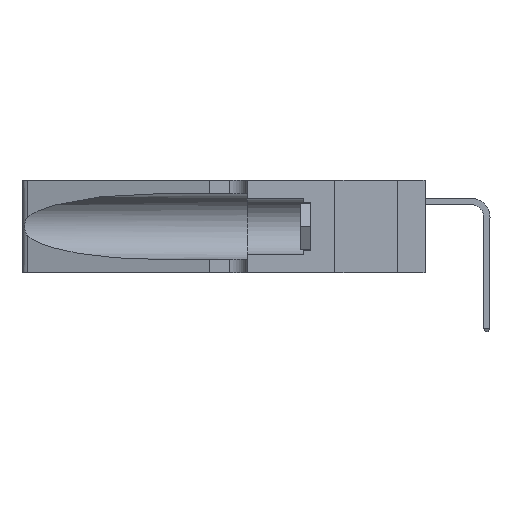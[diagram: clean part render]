
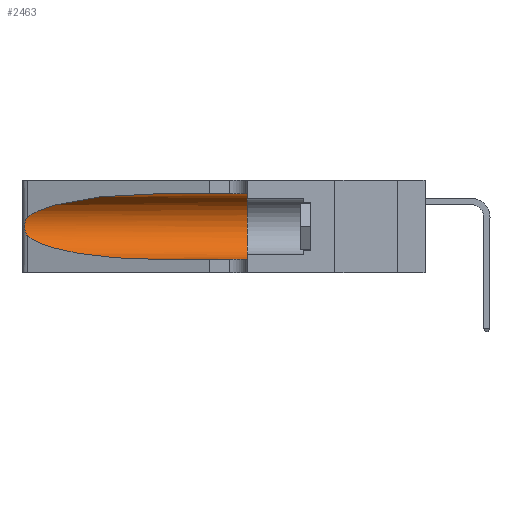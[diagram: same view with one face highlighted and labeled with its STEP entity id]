
A CAD part, left-side view. The second image highlights one B-rep face of the part: STEP entity #2463.
In plain terms, the highlighted cylindrical face has radius 3.308 mm (diameter 6.617 mm), a partial arc.
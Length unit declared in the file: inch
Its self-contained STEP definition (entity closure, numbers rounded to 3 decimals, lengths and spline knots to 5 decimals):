
#19 = EDGE_CURVE ( 'NONE', #4897, #9281, #9336, .T. ) ;
#1151 = CARTESIAN_POINT ( 'NONE',  ( 0.1305, 0.72297, 0.31525 ) ) ;
#1165 = EDGE_CURVE ( 'NONE', #18363, #14374, #10308, .T. ) ;
#2083 = CARTESIAN_POINT ( 'NONE',  ( 0.25487, 1.22718, 0.14631 ) ) ;
#2425 = VECTOR ( 'NONE', #9149, 39.37008 ) ;
#2463 = ADVANCED_FACE ( 'NONE', ( #28487 ), #27783, .F. ) ;
#2698 =( BOUNDED_CURVE ( )  B_SPLINE_CURVE ( 3, ( #21450, #7989, #10233, #25913 ),
 .UNSPECIFIED., .F., .T. ) 
 B_SPLINE_CURVE_WITH_KNOTS ( ( 4, 4 ),
 ( 3.44316, 4.71239 ),
 .UNSPECIFIED. ) 
 CURVE ( )  GEOMETRIC_REPRESENTATION_ITEM ( )  RATIONAL_B_SPLINE_CURVE ( ( 1., 0.87, 0.87, 1. ) ) 
 REPRESENTATION_ITEM ( '' )  );
#3135 = LINE ( 'NONE', #20375, #2425 ) ;
#4897 = VERTEX_POINT ( 'NONE', #9453 ) ;
#5233 = ORIENTED_EDGE ( 'NONE', *, *, #1165, .T. ) ;
#5377 = CARTESIAN_POINT ( 'NONE',  ( 0.25787, 1.23484, 0.2124 ) ) ;
#5499 = CARTESIAN_POINT ( 'NONE',  ( 0.26018, 1.23835, 0.19895 ) ) ;
#6035 = CARTESIAN_POINT ( 'NONE',  ( 0.25487, 1.22718, 0.22369 ) ) ;
#6212 = CARTESIAN_POINT ( 'NONE',  ( 0.1305, 0.35, 0.05475 ) ) ;
#6290 = DIRECTION ( 'NONE',  ( 0., 1., 0. ) ) ;
#6357 = ORIENTED_EDGE ( 'NONE', *, *, #15109, .T. ) ;
#7962 = CARTESIAN_POINT ( 'NONE',  ( 0.2373, 1.15595, 0.28018 ) ) ;
#7989 = CARTESIAN_POINT ( 'NONE',  ( 0.2373, 1.15595, 0.08982 ) ) ;
#8105 = EDGE_CURVE ( 'NONE', #29033, #28754, #3135, .T. ) ;
#8364 = DIRECTION ( 'NONE',  ( 0., -1., 0. ) ) ;
#9149 = DIRECTION ( 'NONE',  ( 0., -1., 0. ) ) ;
#9281 = VERTEX_POINT ( 'NONE', #2083 ) ;
#9336 = B_SPLINE_CURVE_WITH_KNOTS ( 'NONE', 3,
 ( #6035, #24203, #21112, #5377, #25054, #5499, #20204, #19311, #28400, #12207, #18271, #28893, #12236, #26032 ),
 .UNSPECIFIED., .F., .F.,
 ( 4, 2, 2, 2, 2, 2, 4 ),
 ( 0., 0.00027, 0.00053, 0.00107, 0.0016, 0.00187, 0.00214 ),
 .UNSPECIFIED. ) ;
#9420 = CARTESIAN_POINT ( 'NONE',  ( 0.1305, 0.35, 0.31525 ) ) ;
#9453 = CARTESIAN_POINT ( 'NONE',  ( 0.25487, 1.22718, 0.22369 ) ) ;
#10233 = CARTESIAN_POINT ( 'NONE',  ( 0.18966, 0.96281, 0.05475 ) ) ;
#10308 = LINE ( 'NONE', #19622, #16332 ) ;
#10312 = AXIS2_PLACEMENT_3D ( 'NONE', #19779, #6290, #22014 ) ;
#10639 = DIRECTION ( 'NONE',  ( 0., 0., -1. ) ) ;
#10972 =( BOUNDED_CURVE ( )  B_SPLINE_CURVE ( 3, ( #1151, #14653, #7962, #23666 ),
 .UNSPECIFIED., .F., .F. ) 
 B_SPLINE_CURVE_WITH_KNOTS ( ( 4, 4 ),
 ( 1.5708, 2.84003 ),
 .UNSPECIFIED. ) 
 CURVE ( )  GEOMETRIC_REPRESENTATION_ITEM ( )  RATIONAL_B_SPLINE_CURVE ( ( 1., 0.87, 0.87, 1. ) ) 
 REPRESENTATION_ITEM ( '' )  );
#11423 = AXIS2_PLACEMENT_3D ( 'NONE', #19651, #21858, #10639 ) ;
#12207 = CARTESIAN_POINT ( 'NONE',  ( 0.25856, 1.23593, 0.16098 ) ) ;
#12236 = CARTESIAN_POINT ( 'NONE',  ( 0.25555, 1.22993, 0.14849 ) ) ;
#12429 = ORIENTED_EDGE ( 'NONE', *, *, #8105, .F. ) ;
#14333 = ORIENTED_EDGE ( 'NONE', *, *, #19, .T. ) ;
#14374 = VERTEX_POINT ( 'NONE', #6212 ) ;
#14653 = CARTESIAN_POINT ( 'NONE',  ( 0.18966, 0.96281, 0.31525 ) ) ;
#15109 = EDGE_CURVE ( 'NONE', #9281, #18363, #2698, .T. ) ;
#15769 = CARTESIAN_POINT ( 'NONE',  ( 0.1305, 0.72297, 0.05475 ) ) ;
#16332 = VECTOR ( 'NONE', #8364, 39.37008 ) ;
#17617 = EDGE_CURVE ( 'NONE', #29033, #4897, #10972, .T. ) ;
#17755 = EDGE_LOOP ( 'NONE', ( #17910, #14333, #6357, #5233, #22226, #12429 ) ) ;
#17910 = ORIENTED_EDGE ( 'NONE', *, *, #17617, .T. ) ;
#18271 = CARTESIAN_POINT ( 'NONE',  ( 0.25789, 1.23486, 0.15765 ) ) ;
#18363 = VERTEX_POINT ( 'NONE', #15769 ) ;
#18863 = EDGE_CURVE ( 'NONE', #28754, #14374, #26099, .T. ) ;
#19311 = CARTESIAN_POINT ( 'NONE',  ( 0.26075, 1.23896, 0.178 ) ) ;
#19622 = CARTESIAN_POINT ( 'NONE',  ( 0.1305, 1.61858, 0.05475 ) ) ;
#19651 = CARTESIAN_POINT ( 'NONE',  ( 0.1305, 1.61858, 0.185 ) ) ;
#19779 = CARTESIAN_POINT ( 'NONE',  ( 0.1305, 0.35, 0.185 ) ) ;
#20204 = CARTESIAN_POINT ( 'NONE',  ( 0.26075, 1.23896, 0.19203 ) ) ;
#20375 = CARTESIAN_POINT ( 'NONE',  ( 0.1305, 1.61858, 0.31525 ) ) ;
#21112 = CARTESIAN_POINT ( 'NONE',  ( 0.25639, 1.23184, 0.21858 ) ) ;
#21450 = CARTESIAN_POINT ( 'NONE',  ( 0.25487, 1.22718, 0.14631 ) ) ;
#21858 = DIRECTION ( 'NONE',  ( 0., -1., 0. ) ) ;
#22014 = DIRECTION ( 'NONE',  ( 0., 0., 1. ) ) ;
#22226 = ORIENTED_EDGE ( 'NONE', *, *, #18863, .F. ) ;
#23666 = CARTESIAN_POINT ( 'NONE',  ( 0.25487, 1.22718, 0.22369 ) ) ;
#24203 = CARTESIAN_POINT ( 'NONE',  ( 0.25555, 1.22994, 0.2215 ) ) ;
#25054 = CARTESIAN_POINT ( 'NONE',  ( 0.25854, 1.2359, 0.20912 ) ) ;
#25913 = CARTESIAN_POINT ( 'NONE',  ( 0.1305, 0.72297, 0.05475 ) ) ;
#26032 = CARTESIAN_POINT ( 'NONE',  ( 0.25487, 1.22718, 0.14631 ) ) ;
#26054 = CARTESIAN_POINT ( 'NONE',  ( 0.1305, 0.72297, 0.31525 ) ) ;
#26099 = CIRCLE ( 'NONE', #10312, 0.13025 ) ;
#27783 = CYLINDRICAL_SURFACE ( 'NONE', #11423, 0.13025 ) ;
#28400 = CARTESIAN_POINT ( 'NONE',  ( 0.26017, 1.23833, 0.17102 ) ) ;
#28487 = FACE_OUTER_BOUND ( 'NONE', #17755, .T. ) ;
#28754 = VERTEX_POINT ( 'NONE', #9420 ) ;
#28893 = CARTESIAN_POINT ( 'NONE',  ( 0.25639, 1.23186, 0.15144 ) ) ;
#29033 = VERTEX_POINT ( 'NONE', #26054 ) ;
